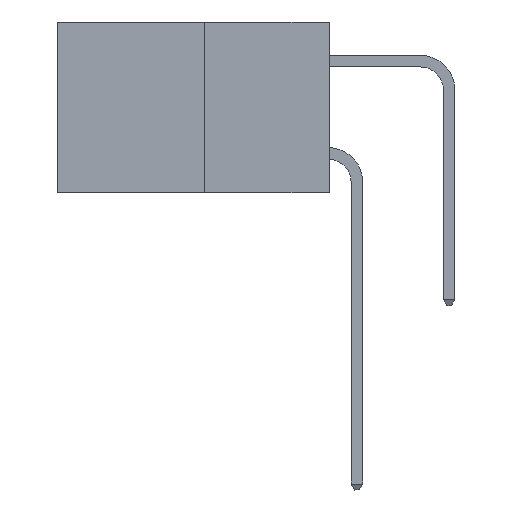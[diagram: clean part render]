
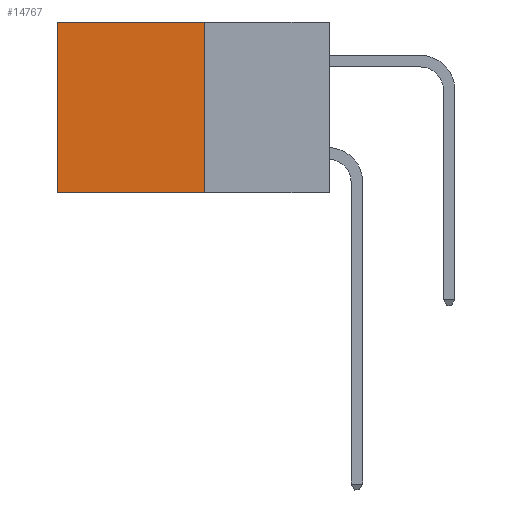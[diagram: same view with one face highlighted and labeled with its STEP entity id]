
A CAD part, left-side view. The second image highlights one B-rep face of the part: STEP entity #14767.
In plain terms, the highlighted planar face has unit normal (-1, 0, 0).
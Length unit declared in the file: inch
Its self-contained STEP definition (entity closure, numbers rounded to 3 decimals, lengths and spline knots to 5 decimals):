
#6 = EDGE_CURVE ( 'NONE', #13287, #11315, #20961, .T. ) ;
#1307 = PLANE ( 'NONE',  #16528 ) ;
#1569 = EDGE_CURVE ( 'NONE', #7965, #22200, #8142, .T. ) ;
#1749 = LINE ( 'NONE', #2385, #6158 ) ;
#2385 = CARTESIAN_POINT ( 'NONE',  ( 0.277, 0.27, -0.37 ) ) ;
#2981 = CARTESIAN_POINT ( 'NONE',  ( 0.277, 0.27, 0. ) ) ;
#3858 = DIRECTION ( 'NONE',  ( 0., 1., 0. ) ) ;
#4465 = CARTESIAN_POINT ( 'NONE',  ( 0.277, 0.27, -0.37 ) ) ;
#6158 = VECTOR ( 'NONE', #3858, 39.37008 ) ;
#7965 = VERTEX_POINT ( 'NONE', #9614 ) ;
#8142 = LINE ( 'NONE', #15522, #11905 ) ;
#8448 = EDGE_CURVE ( 'NONE', #22200, #11315, #1749, .T. ) ;
#8696 = EDGE_CURVE ( 'NONE', #7965, #13287, #20029, .T. ) ;
#9614 = CARTESIAN_POINT ( 'NONE',  ( 0.277, 0.27, 0. ) ) ;
#10521 = ORIENTED_EDGE ( 'NONE', *, *, #6, .T. ) ;
#10693 = DIRECTION ( 'NONE',  ( 1., 0., 0. ) ) ;
#11315 = VERTEX_POINT ( 'NONE', #14441 ) ;
#11905 = VECTOR ( 'NONE', #17419, 39.37008 ) ;
#13128 = ORIENTED_EDGE ( 'NONE', *, *, #1569, .F. ) ;
#13287 = VERTEX_POINT ( 'NONE', #17790 ) ;
#13829 = FACE_OUTER_BOUND ( 'NONE', #16689, .T. ) ;
#14441 = CARTESIAN_POINT ( 'NONE',  ( 0.277, 0.59, -0.37 ) ) ;
#14767 = ADVANCED_FACE ( 'NONE', ( #13829 ), #1307, .F. ) ;
#15093 = VECTOR ( 'NONE', #19647, 39.37008 ) ;
#15522 = CARTESIAN_POINT ( 'NONE',  ( 0.277, 0.27, -0.37 ) ) ;
#15992 = VECTOR ( 'NONE', #16315, 39.37008 ) ;
#16315 = DIRECTION ( 'NONE',  ( 0., 0., -1. ) ) ;
#16528 = AXIS2_PLACEMENT_3D ( 'NONE', #21788, #10693, #23638 ) ;
#16689 = EDGE_LOOP ( 'NONE', ( #10521, #18530, #13128, #18128 ) ) ;
#17419 = DIRECTION ( 'NONE',  ( 0., 0., -1. ) ) ;
#17790 = CARTESIAN_POINT ( 'NONE',  ( 0.277, 0.59, 0. ) ) ;
#18128 = ORIENTED_EDGE ( 'NONE', *, *, #8696, .T. ) ;
#18530 = ORIENTED_EDGE ( 'NONE', *, *, #8448, .F. ) ;
#19647 = DIRECTION ( 'NONE',  ( 0., 1., 0. ) ) ;
#20029 = LINE ( 'NONE', #2981, #15093 ) ;
#20961 = LINE ( 'NONE', #21190, #15992 ) ;
#21190 = CARTESIAN_POINT ( 'NONE',  ( 0.277, 0.59, -0.37 ) ) ;
#21788 = CARTESIAN_POINT ( 'NONE',  ( 0.277, 0.27, -0.37 ) ) ;
#22200 = VERTEX_POINT ( 'NONE', #4465 ) ;
#23638 = DIRECTION ( 'NONE',  ( 0., 0., -1. ) ) ;
